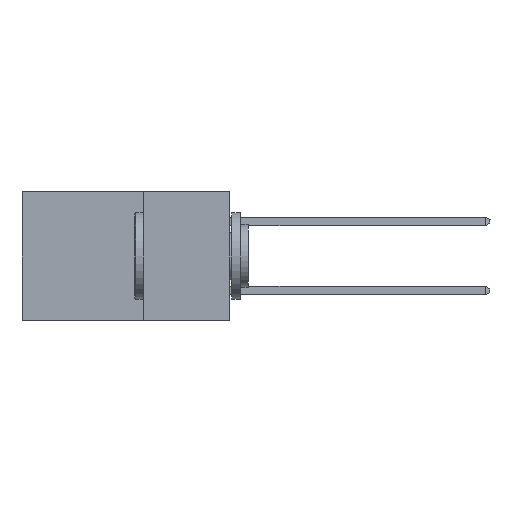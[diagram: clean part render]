
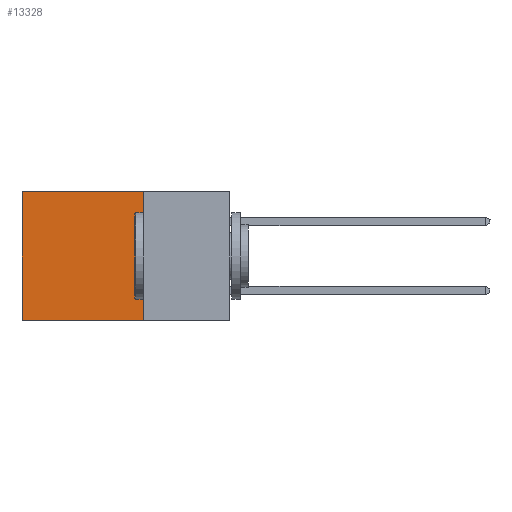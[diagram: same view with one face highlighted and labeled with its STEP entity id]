
A CAD part, left-side view. The second image highlights one B-rep face of the part: STEP entity #13328.
In plain terms, the highlighted planar face has unit normal (-1, 0, 0).
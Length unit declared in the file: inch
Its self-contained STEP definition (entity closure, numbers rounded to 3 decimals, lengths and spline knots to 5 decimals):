
#323 = PLANE ( 'NONE',  #2939 ) ;
#528 = VERTEX_POINT ( 'NONE', #7684 ) ;
#537 = CARTESIAN_POINT ( 'NONE',  ( 0.2615, 0.6, -0.37 ) ) ;
#1237 = CARTESIAN_POINT ( 'NONE',  ( 0.2615, 0.25, -0.37 ) ) ;
#1463 = EDGE_LOOP ( 'NONE', ( #2691, #4877, #1669, #8219 ) ) ;
#1592 = CARTESIAN_POINT ( 'NONE',  ( 0.2615, 0.6, -0.37 ) ) ;
#1617 = FACE_OUTER_BOUND ( 'NONE', #1463, .T. ) ;
#1669 = ORIENTED_EDGE ( 'NONE', *, *, #4383, .F. ) ;
#1753 = LINE ( 'NONE', #1592, #7166 ) ;
#1770 = CARTESIAN_POINT ( 'NONE',  ( 0.2615, 0.25, -0.37 ) ) ;
#2691 = ORIENTED_EDGE ( 'NONE', *, *, #10373, .T. ) ;
#2939 = AXIS2_PLACEMENT_3D ( 'NONE', #6453, #10014, #9778 ) ;
#3236 = CARTESIAN_POINT ( 'NONE',  ( 0.2615, 0.25, 0. ) ) ;
#4383 = EDGE_CURVE ( 'NONE', #528, #5556, #12105, .T. ) ;
#4877 = ORIENTED_EDGE ( 'NONE', *, *, #6953, .F. ) ;
#5556 = VERTEX_POINT ( 'NONE', #7760 ) ;
#5588 = VERTEX_POINT ( 'NONE', #537 ) ;
#5598 = VECTOR ( 'NONE', #7969, 39.37008 ) ;
#5642 = VECTOR ( 'NONE', #7865, 39.37008 ) ;
#6453 = CARTESIAN_POINT ( 'NONE',  ( 0.2615, 0.25, -0.37 ) ) ;
#6588 = DIRECTION ( 'NONE',  ( 0., 0., -1. ) ) ;
#6879 = VERTEX_POINT ( 'NONE', #14928 ) ;
#6953 = EDGE_CURVE ( 'NONE', #5556, #5588, #8665, .T. ) ;
#7166 = VECTOR ( 'NONE', #6588, 39.37008 ) ;
#7684 = CARTESIAN_POINT ( 'NONE',  ( 0.2615, 0.25, 0. ) ) ;
#7760 = CARTESIAN_POINT ( 'NONE',  ( 0.2615, 0.25, -0.37 ) ) ;
#7865 = DIRECTION ( 'NONE',  ( 0., 1., 0. ) ) ;
#7969 = DIRECTION ( 'NONE',  ( 0., 0., -1. ) ) ;
#8061 = DIRECTION ( 'NONE',  ( 0., 1., 0. ) ) ;
#8219 = ORIENTED_EDGE ( 'NONE', *, *, #15103, .T. ) ;
#8665 = LINE ( 'NONE', #1770, #5642 ) ;
#9778 = DIRECTION ( 'NONE',  ( 0., 0., -1. ) ) ;
#10014 = DIRECTION ( 'NONE',  ( 1., 0., 0. ) ) ;
#10373 = EDGE_CURVE ( 'NONE', #6879, #5588, #1753, .T. ) ;
#12105 = LINE ( 'NONE', #1237, #5598 ) ;
#13328 = ADVANCED_FACE ( 'NONE', ( #1617 ), #323, .F. ) ;
#14087 = LINE ( 'NONE', #3236, #14335 ) ;
#14335 = VECTOR ( 'NONE', #8061, 39.37008 ) ;
#14928 = CARTESIAN_POINT ( 'NONE',  ( 0.2615, 0.6, 0. ) ) ;
#15103 = EDGE_CURVE ( 'NONE', #528, #6879, #14087, .T. ) ;
